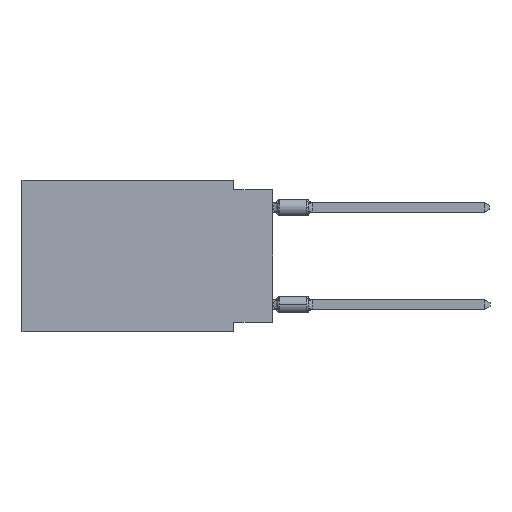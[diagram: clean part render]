
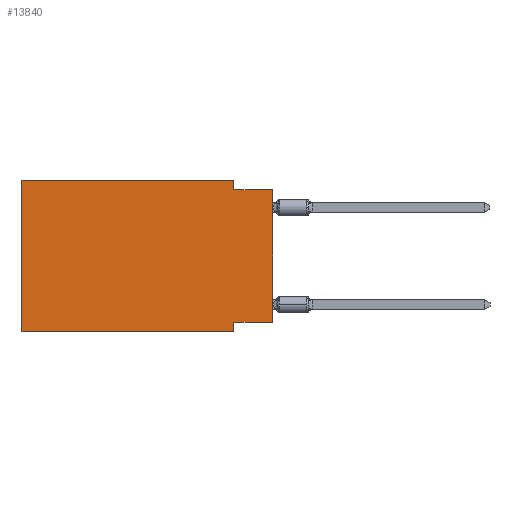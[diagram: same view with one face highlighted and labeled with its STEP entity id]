
A CAD part, left-side view. The second image highlights one B-rep face of the part: STEP entity #13840.
In plain terms, the highlighted planar face has unit normal (-1, 0, 0).
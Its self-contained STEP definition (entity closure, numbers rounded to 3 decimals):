
#25 = CARTESIAN_POINT ( 'NONE',  ( 0., 16.383, 0. ) ) ;
#1111 = EDGE_CURVE ( 'NONE', #17200, #20992, #1786, .T. ) ;
#1332 = VERTEX_POINT ( 'NONE', #21363 ) ;
#1786 = LINE ( 'NONE', #13753, #5863 ) ;
#3645 = VECTOR ( 'NONE', #16227, 1000. ) ;
#4030 = CARTESIAN_POINT ( 'NONE',  ( 0., 2.54, -9.271 ) ) ;
#4741 = CARTESIAN_POINT ( 'NONE',  ( 0., 0., -0.635 ) ) ;
#5554 = VERTEX_POINT ( 'NONE', #19341 ) ;
#5863 = VECTOR ( 'NONE', #8816, 1000. ) ;
#6155 = ORIENTED_EDGE ( 'NONE', *, *, #16507, .F. ) ;
#6629 = VERTEX_POINT ( 'NONE', #9935 ) ;
#6895 = EDGE_CURVE ( 'NONE', #5554, #17469, #14020, .T. ) ;
#7162 = DIRECTION ( 'NONE',  ( 0., -1., 0. ) ) ;
#7320 = VECTOR ( 'NONE', #11509, 1000. ) ;
#7688 = CARTESIAN_POINT ( 'NONE',  ( 0., 16.383, 0. ) ) ;
#8307 = PLANE ( 'NONE',  #19889 ) ;
#8564 = LINE ( 'NONE', #25, #11785 ) ;
#8816 = DIRECTION ( 'NONE',  ( 0., 0., -1. ) ) ;
#9206 = CARTESIAN_POINT ( 'NONE',  ( 0., 16.383, -9.906 ) ) ;
#9831 = CARTESIAN_POINT ( 'NONE',  ( 0., 16.383, 0. ) ) ;
#9935 = CARTESIAN_POINT ( 'NONE',  ( 0., 16.383, -9.906 ) ) ;
#10029 = DIRECTION ( 'NONE',  ( 0., 0., -1. ) ) ;
#10040 = ORIENTED_EDGE ( 'NONE', *, *, #13457, .T. ) ;
#10053 = CARTESIAN_POINT ( 'NONE',  ( 0., 0., 0. ) ) ;
#10073 = ORIENTED_EDGE ( 'NONE', *, *, #6895, .F. ) ;
#11509 = DIRECTION ( 'NONE',  ( 0., -1., 0. ) ) ;
#11546 = LINE ( 'NONE', #18583, #20612 ) ;
#11785 = VECTOR ( 'NONE', #7162, 1000. ) ;
#11885 = DIRECTION ( 'NONE',  ( 0., 0., 1. ) ) ;
#11887 = LINE ( 'NONE', #10053, #22398 ) ;
#12121 = EDGE_CURVE ( 'NONE', #17469, #16899, #13357, .T. ) ;
#12389 = EDGE_CURVE ( 'NONE', #6629, #20992, #17840, .T. ) ;
#12635 = CARTESIAN_POINT ( 'NONE',  ( 0., 2.54, 0. ) ) ;
#13357 = LINE ( 'NONE', #18545, #7320 ) ;
#13457 = EDGE_CURVE ( 'NONE', #1332, #16899, #11887, .T. ) ;
#13518 = EDGE_CURVE ( 'NONE', #1332, #17200, #11546, .T. ) ;
#13545 = EDGE_CURVE ( 'NONE', #22475, #5554, #8564, .T. ) ;
#13753 = CARTESIAN_POINT ( 'NONE',  ( 0., 2.54, -9.906 ) ) ;
#13840 = ADVANCED_FACE ( 'NONE', ( #14863 ), #8307, .F. ) ;
#14020 = LINE ( 'NONE', #12635, #14888 ) ;
#14863 = FACE_OUTER_BOUND ( 'NONE', #19501, .T. ) ;
#14888 = VECTOR ( 'NONE', #17823, 1000. ) ;
#16036 = DIRECTION ( 'NONE',  ( 0., 1., 0. ) ) ;
#16227 = DIRECTION ( 'NONE',  ( 0., -1., 0. ) ) ;
#16507 = EDGE_CURVE ( 'NONE', #6629, #22475, #18817, .T. ) ;
#16869 = ORIENTED_EDGE ( 'NONE', *, *, #1111, .F. ) ;
#16899 = VERTEX_POINT ( 'NONE', #4741 ) ;
#17129 = VECTOR ( 'NONE', #11885, 1000. ) ;
#17200 = VERTEX_POINT ( 'NONE', #4030 ) ;
#17469 = VERTEX_POINT ( 'NONE', #19980 ) ;
#17823 = DIRECTION ( 'NONE',  ( 0., 0., -1. ) ) ;
#17840 = LINE ( 'NONE', #9206, #3645 ) ;
#18430 = ORIENTED_EDGE ( 'NONE', *, *, #13518, .F. ) ;
#18545 = CARTESIAN_POINT ( 'NONE',  ( 0., 0., -0.635 ) ) ;
#18583 = CARTESIAN_POINT ( 'NONE',  ( 0., 0., -9.271 ) ) ;
#18817 = LINE ( 'NONE', #9831, #17129 ) ;
#18819 = DIRECTION ( 'NONE',  ( 0., 0., 1. ) ) ;
#18861 = ORIENTED_EDGE ( 'NONE', *, *, #13545, .F. ) ;
#19341 = CARTESIAN_POINT ( 'NONE',  ( 0., 2.54, 0. ) ) ;
#19501 = EDGE_LOOP ( 'NONE', ( #10040, #20187, #10073, #18861, #6155, #22392, #16869, #18430 ) ) ;
#19889 = AXIS2_PLACEMENT_3D ( 'NONE', #22016, #20182, #10029 ) ;
#19980 = CARTESIAN_POINT ( 'NONE',  ( 0., 2.54, -0.635 ) ) ;
#20182 = DIRECTION ( 'NONE',  ( 1., 0., 0. ) ) ;
#20187 = ORIENTED_EDGE ( 'NONE', *, *, #12121, .F. ) ;
#20612 = VECTOR ( 'NONE', #16036, 1000. ) ;
#20992 = VERTEX_POINT ( 'NONE', #22549 ) ;
#21363 = CARTESIAN_POINT ( 'NONE',  ( 0., 0., -9.271 ) ) ;
#22016 = CARTESIAN_POINT ( 'NONE',  ( 0., 16.383, 0. ) ) ;
#22392 = ORIENTED_EDGE ( 'NONE', *, *, #12389, .T. ) ;
#22398 = VECTOR ( 'NONE', #18819, 1000. ) ;
#22475 = VERTEX_POINT ( 'NONE', #7688 ) ;
#22549 = CARTESIAN_POINT ( 'NONE',  ( 0., 2.54, -9.906 ) ) ;
